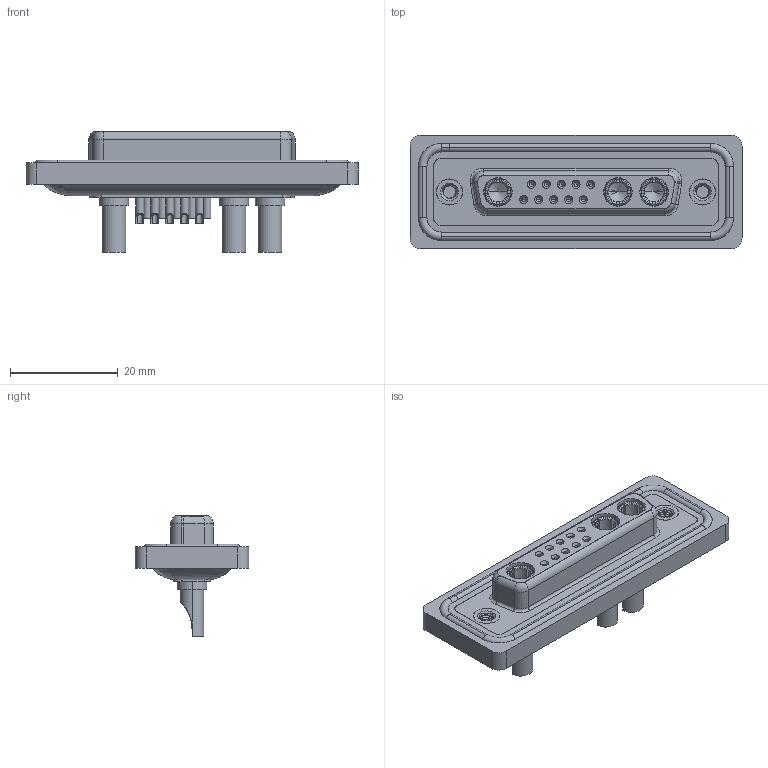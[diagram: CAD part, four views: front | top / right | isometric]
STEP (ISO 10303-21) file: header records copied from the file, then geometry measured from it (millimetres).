
FILE_DESCRIPTION (( 'STEP AP203' ), '1' );
FILE_NAME ('628W13W3322-3NA.STEP', '2024-04-09T20:29:39', ( '' ), ( '' ), 'SwSTEP 2.0', 'SolidWorks 2023', '' );
FILE_SCHEMA (( 'CONFIG_CONTROL_DESIGN' ));
Length unit declared in the file: millimetre
Products named in the file (9): 628W13W3322-3NA; 628Combo Threaded Rivet_A; Power Socket_30A SC; 628Combo Contact Row 1_22; 628Combo Waterproof Housing_25 Contacts; 628Combo Shell Rear_25 Contacts; 628Combo Housing_13W3; 628Combo Shell Front_25 Contacts; 628Combo Contact Row 2_22
Assembly tree (19 placements, depth 2):
  628W13W3322-3NA
    628Combo Housing_13W3
    628Combo Waterproof Housing_25 Contacts
    628Combo Shell Front_25 Contacts
    628Combo Shell Rear_25 Contacts
    628Combo Threaded Rivet_A  x2
    628Combo Contact Row 1_22  x5
    628Combo Contact Row 2_22  x5
    Power Socket_30A SC  x3
Bounding box: 61.75 x 21.1 x 22.45 mm (x, y, z)
Volume: 8367.3 mm3; surface area: 14133.9 mm2
Topology: 23 solids, 23 shells, 1174 faces, 2958 edges, 1850 vertices
Faces by surface type: cylinder 478, plane 371, torus 163, cone 149, bspline 13
Entity records: 23103 total; most frequent: CARTESIAN_POINT 6033, DIRECTION 3530, ORIENTED_EDGE 3192, EDGE_CURVE 1596, AXIS2_PLACEMENT_3D 1437, VERTEX_POINT 1016, CIRCLE 767, EDGE_LOOP 754
